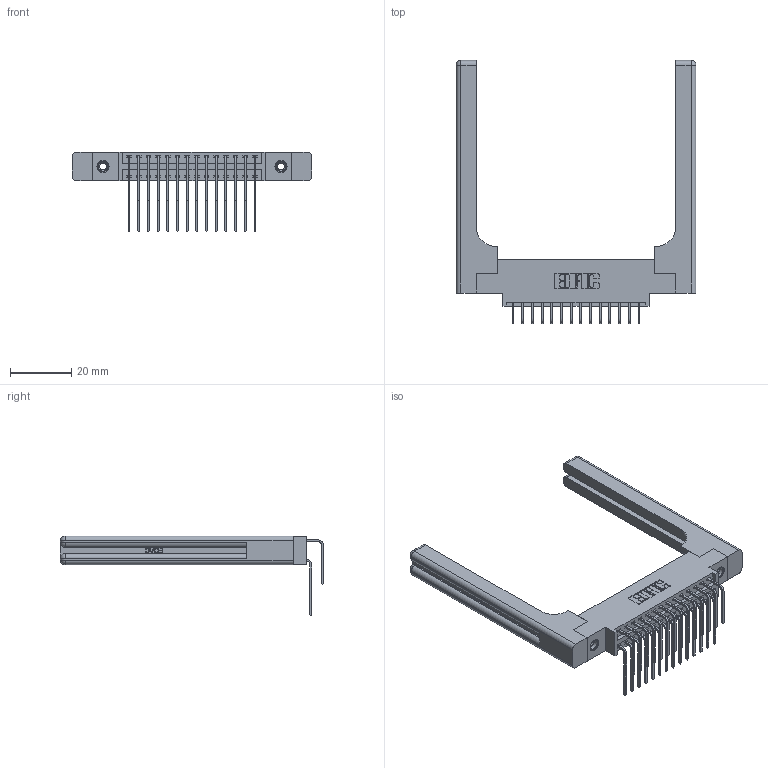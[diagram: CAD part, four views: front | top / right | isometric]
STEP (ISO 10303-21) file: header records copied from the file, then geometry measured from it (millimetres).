
FILE_DESCRIPTION (( 'STEP AP203' ), '1' );
FILE_NAME ('346-028-559-858.STEP', '2022-05-19T15:43:41', ( '' ), ( '' ), 'SwSTEP 2.0', 'SolidWorks 2020', '' );
FILE_SCHEMA (( 'CONFIG_CONTROL_DESIGN' ));
Length unit declared in the file: inch
Products named in the file (6): 345-292-001_559 Tail - 2; 346 Part_0.170 Offset - 0.156 Dia-TH; 345-292-001_558 559 Tail - 1; 346-220-058_345-220-058; 346-028-559-858; 345-250-001_345-250-001-102
Assembly tree (33 placements, depth 2):
  346-028-559-858
    346 Part_0.170 Offset - 0.156 Dia-TH
    345-292-001_558 559 Tail - 1  x14
    345-292-001_559 Tail - 2  x14
    345-250-001_345-250-001-102  x2
    346-220-058_345-220-058  x2
Bounding box: 78.51 x 86.17 x 26.16 mm (x, y, z)
Volume: 14921.4 mm3; surface area: 15730.9 mm2
Topology: 33 solids, 33 shells, 1908 faces, 5551 edges, 3642 vertices
Faces by surface type: plane 1278, cylinder 570, bspline 36, cone 12, sphere 8, torus 4
Entity records: 20420 total; most frequent: CARTESIAN_POINT 4470, ORIENTED_EDGE 3148, DIRECTION 2894, EDGE_CURVE 1574, LINE 1254, VECTOR 1254, VERTEX_POINT 1038, AXIS2_PLACEMENT_3D 820
